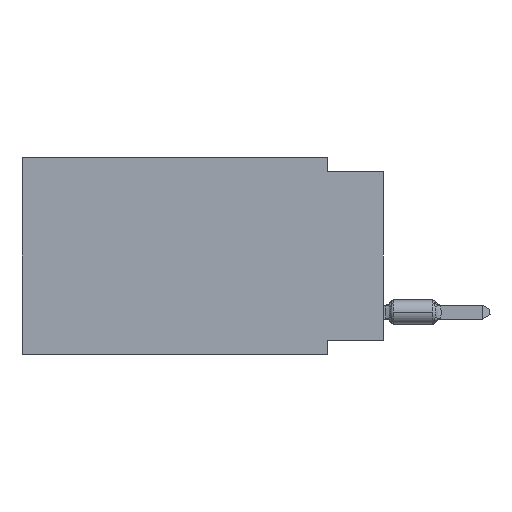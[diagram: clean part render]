
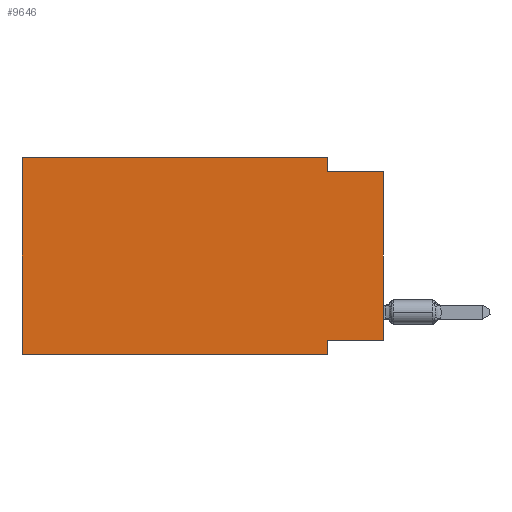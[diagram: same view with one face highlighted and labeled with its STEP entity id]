
A CAD part, left-side view. The second image highlights one B-rep face of the part: STEP entity #9646.
In plain terms, the highlighted planar face has unit normal (-1, 0, 0).
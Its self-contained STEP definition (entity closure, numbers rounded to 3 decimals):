
#1081 = ORIENTED_EDGE ( 'NONE', *, *, #11313, .T. ) ;
#1604 = VECTOR ( 'NONE', #14077, 1000. ) ;
#1867 = LINE ( 'NONE', #10664, #6604 ) ;
#3266 = VECTOR ( 'NONE', #16047, 1000. ) ;
#4328 = VERTEX_POINT ( 'NONE', #13061 ) ;
#4510 = ORIENTED_EDGE ( 'NONE', *, *, #7959, .T. ) ;
#4660 = VERTEX_POINT ( 'NONE', #19072 ) ;
#4895 = LINE ( 'NONE', #7320, #12122 ) ;
#5023 = CARTESIAN_POINT ( 'NONE',  ( 0., 2.54, -8.89 ) ) ;
#5307 = ORIENTED_EDGE ( 'NONE', *, *, #7721, .F. ) ;
#5367 = DIRECTION ( 'NONE',  ( 0., -1., 0. ) ) ;
#5447 = CARTESIAN_POINT ( 'NONE',  ( 0., 2.54, -8.89 ) ) ;
#5568 = CARTESIAN_POINT ( 'NONE',  ( 0., 16.383, 0. ) ) ;
#6168 = LINE ( 'NONE', #21428, #10473 ) ;
#6604 = VECTOR ( 'NONE', #10805, 1000. ) ;
#6797 = CARTESIAN_POINT ( 'NONE',  ( 0., 2.54, -0.635 ) ) ;
#7320 = CARTESIAN_POINT ( 'NONE',  ( 0., 16.383, -8.89 ) ) ;
#7721 = EDGE_CURVE ( 'NONE', #4328, #27847, #1867, .T. ) ;
#7959 = EDGE_CURVE ( 'NONE', #4328, #11067, #4895, .T. ) ;
#8208 = VERTEX_POINT ( 'NONE', #17618 ) ;
#9646 = ADVANCED_FACE ( 'NONE', ( #27427 ), #25270, .F. ) ;
#10013 = VECTOR ( 'NONE', #5367, 1000. ) ;
#10473 = VECTOR ( 'NONE', #10641, 1000. ) ;
#10641 = DIRECTION ( 'NONE',  ( 0., 0., -1. ) ) ;
#10664 = CARTESIAN_POINT ( 'NONE',  ( 0., 16.383, 0. ) ) ;
#10805 = DIRECTION ( 'NONE',  ( 0., 0., 1. ) ) ;
#11067 = VERTEX_POINT ( 'NONE', #5023 ) ;
#11313 = EDGE_CURVE ( 'NONE', #14712, #12715, #17935, .T. ) ;
#11507 = EDGE_LOOP ( 'NONE', ( #1081, #14888, #27240, #23901, #5307, #4510, #13382, #13521 ) ) ;
#11854 = CARTESIAN_POINT ( 'NONE',  ( 0., 16.383, 0. ) ) ;
#12122 = VECTOR ( 'NONE', #13392, 1000. ) ;
#12715 = VERTEX_POINT ( 'NONE', #16903 ) ;
#13061 = CARTESIAN_POINT ( 'NONE',  ( 0., 16.383, -8.89 ) ) ;
#13255 = VERTEX_POINT ( 'NONE', #6797 ) ;
#13382 = ORIENTED_EDGE ( 'NONE', *, *, #23798, .F. ) ;
#13392 = DIRECTION ( 'NONE',  ( 0., -1., 0. ) ) ;
#13521 = ORIENTED_EDGE ( 'NONE', *, *, #16341, .F. ) ;
#13616 = CARTESIAN_POINT ( 'NONE',  ( 0., 0., 0. ) ) ;
#13723 = CARTESIAN_POINT ( 'NONE',  ( 0., 0., -0.635 ) ) ;
#14067 = EDGE_CURVE ( 'NONE', #8208, #13255, #6168, .T. ) ;
#14077 = DIRECTION ( 'NONE',  ( 0., 0., -1. ) ) ;
#14430 = LINE ( 'NONE', #11854, #10013 ) ;
#14712 = VERTEX_POINT ( 'NONE', #25632 ) ;
#14888 = ORIENTED_EDGE ( 'NONE', *, *, #21854, .F. ) ;
#15241 = LINE ( 'NONE', #25885, #24691 ) ;
#16047 = DIRECTION ( 'NONE',  ( 0., 0., 1. ) ) ;
#16341 = EDGE_CURVE ( 'NONE', #14712, #4660, #15241, .T. ) ;
#16903 = CARTESIAN_POINT ( 'NONE',  ( 0., 0., -0.635 ) ) ;
#17618 = CARTESIAN_POINT ( 'NONE',  ( 0., 2.54, 0. ) ) ;
#17935 = LINE ( 'NONE', #13616, #3266 ) ;
#18254 = LINE ( 'NONE', #5447, #1604 ) ;
#19072 = CARTESIAN_POINT ( 'NONE',  ( 0., 2.54, -8.255 ) ) ;
#19130 = DIRECTION ( 'NONE',  ( 0., 1., 0. ) ) ;
#19355 = CARTESIAN_POINT ( 'NONE',  ( 0., 16.383, 0. ) ) ;
#20687 = EDGE_CURVE ( 'NONE', #27847, #8208, #14430, .T. ) ;
#20882 = AXIS2_PLACEMENT_3D ( 'NONE', #5568, #25411, #23259 ) ;
#21428 = CARTESIAN_POINT ( 'NONE',  ( 0., 2.54, 0. ) ) ;
#21854 = EDGE_CURVE ( 'NONE', #13255, #12715, #27225, .T. ) ;
#22505 = DIRECTION ( 'NONE',  ( 0., -1., 0. ) ) ;
#23238 = VECTOR ( 'NONE', #22505, 1000. ) ;
#23259 = DIRECTION ( 'NONE',  ( 0., 0., -1. ) ) ;
#23798 = EDGE_CURVE ( 'NONE', #4660, #11067, #18254, .T. ) ;
#23901 = ORIENTED_EDGE ( 'NONE', *, *, #20687, .F. ) ;
#24691 = VECTOR ( 'NONE', #19130, 1000. ) ;
#25270 = PLANE ( 'NONE',  #20882 ) ;
#25411 = DIRECTION ( 'NONE',  ( 1., 0., 0. ) ) ;
#25632 = CARTESIAN_POINT ( 'NONE',  ( 0., 0., -8.255 ) ) ;
#25885 = CARTESIAN_POINT ( 'NONE',  ( 0., 0., -8.255 ) ) ;
#27225 = LINE ( 'NONE', #13723, #23238 ) ;
#27240 = ORIENTED_EDGE ( 'NONE', *, *, #14067, .F. ) ;
#27427 = FACE_OUTER_BOUND ( 'NONE', #11507, .T. ) ;
#27847 = VERTEX_POINT ( 'NONE', #19355 ) ;
